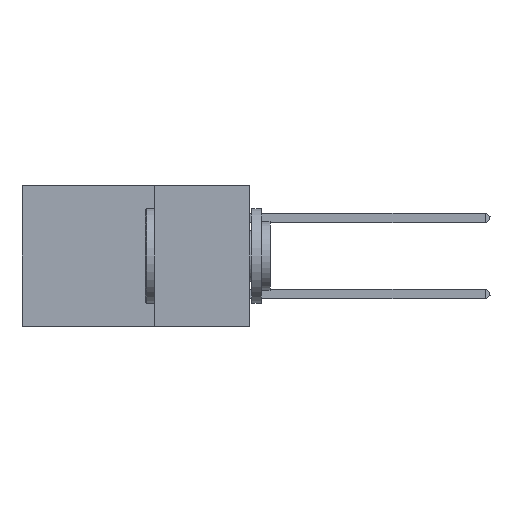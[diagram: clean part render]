
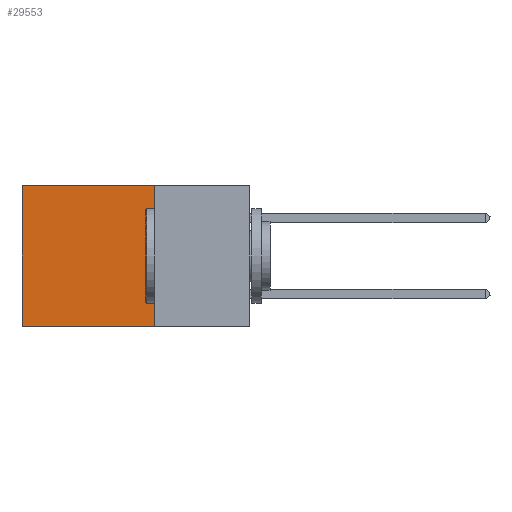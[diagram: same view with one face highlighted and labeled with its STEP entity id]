
A CAD part, left-side view. The second image highlights one B-rep face of the part: STEP entity #29553.
In plain terms, the highlighted planar face has unit normal (-1, 0, 0).
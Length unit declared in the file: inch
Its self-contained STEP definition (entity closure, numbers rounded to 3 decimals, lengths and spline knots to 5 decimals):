
#187 = VECTOR ( 'NONE', #1741, 39.37008 ) ;
#1741 = DIRECTION ( 'NONE',  ( 0., 0., -1. ) ) ;
#3328 = ORIENTED_EDGE ( 'NONE', *, *, #11060, .T. ) ;
#4630 = VECTOR ( 'NONE', #32068, 39.37008 ) ;
#4718 = LINE ( 'NONE', #4820, #18321 ) ;
#4820 = CARTESIAN_POINT ( 'NONE',  ( 0.2875, 0.25, -0.37 ) ) ;
#5017 = ORIENTED_EDGE ( 'NONE', *, *, #32581, .F. ) ;
#5556 = VERTEX_POINT ( 'NONE', #16743 ) ;
#8936 = PLANE ( 'NONE',  #31202 ) ;
#11060 = EDGE_CURVE ( 'NONE', #18925, #31146, #25416, .T. ) ;
#11653 = DIRECTION ( 'NONE',  ( 1., 0., 0. ) ) ;
#11709 = CARTESIAN_POINT ( 'NONE',  ( 0.2875, 0.6, 0. ) ) ;
#12248 = VERTEX_POINT ( 'NONE', #21908 ) ;
#14571 = DIRECTION ( 'NONE',  ( 0., 0., -1. ) ) ;
#14769 = EDGE_CURVE ( 'NONE', #5556, #18925, #26167, .T. ) ;
#16122 = EDGE_LOOP ( 'NONE', ( #3328, #22070, #5017, #21247 ) ) ;
#16743 = CARTESIAN_POINT ( 'NONE',  ( 0.2875, 0.25, 0. ) ) ;
#18321 = VECTOR ( 'NONE', #26397, 39.37008 ) ;
#18925 = VERTEX_POINT ( 'NONE', #11709 ) ;
#21033 = LINE ( 'NONE', #26077, #187 ) ;
#21247 = ORIENTED_EDGE ( 'NONE', *, *, #14769, .T. ) ;
#21908 = CARTESIAN_POINT ( 'NONE',  ( 0.2875, 0.25, -0.37 ) ) ;
#22070 = ORIENTED_EDGE ( 'NONE', *, *, #27830, .F. ) ;
#22559 = CARTESIAN_POINT ( 'NONE',  ( 0.2875, 0.6, 0. ) ) ;
#24597 = VECTOR ( 'NONE', #14571, 39.37008 ) ;
#25038 = CARTESIAN_POINT ( 'NONE',  ( 0.2875, 0.25, 0. ) ) ;
#25416 = LINE ( 'NONE', #22559, #24597 ) ;
#26077 = CARTESIAN_POINT ( 'NONE',  ( 0.2875, 0.25, 0. ) ) ;
#26167 = LINE ( 'NONE', #29367, #4630 ) ;
#26397 = DIRECTION ( 'NONE',  ( 0., 1., 0. ) ) ;
#26458 = CARTESIAN_POINT ( 'NONE',  ( 0.2875, 0.6, -0.37 ) ) ;
#27830 = EDGE_CURVE ( 'NONE', #12248, #31146, #4718, .T. ) ;
#29367 = CARTESIAN_POINT ( 'NONE',  ( 0.2875, 0.25, 0. ) ) ;
#29553 = ADVANCED_FACE ( 'NONE', ( #32397 ), #8936, .F. ) ;
#30410 = DIRECTION ( 'NONE',  ( 0., 0., -1. ) ) ;
#31146 = VERTEX_POINT ( 'NONE', #26458 ) ;
#31202 = AXIS2_PLACEMENT_3D ( 'NONE', #25038, #11653, #30410 ) ;
#32068 = DIRECTION ( 'NONE',  ( 0., 1., 0. ) ) ;
#32397 = FACE_OUTER_BOUND ( 'NONE', #16122, .T. ) ;
#32581 = EDGE_CURVE ( 'NONE', #5556, #12248, #21033, .T. ) ;
